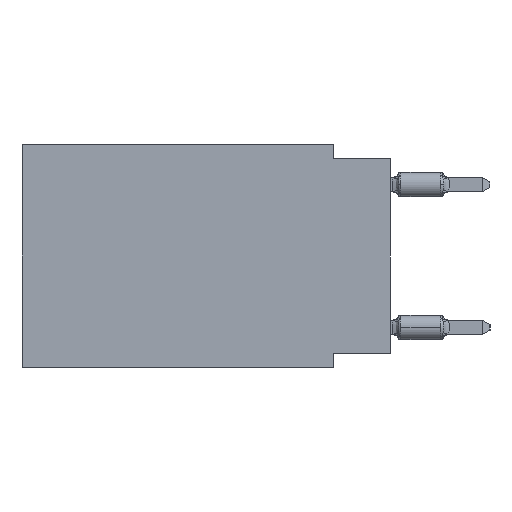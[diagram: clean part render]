
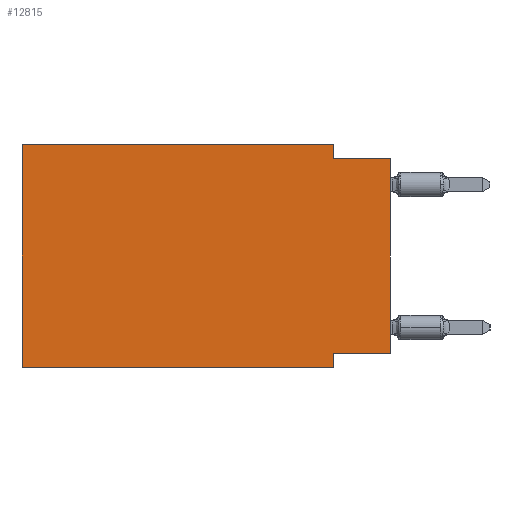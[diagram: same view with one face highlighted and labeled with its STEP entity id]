
A CAD part, left-side view. The second image highlights one B-rep face of the part: STEP entity #12815.
In plain terms, the highlighted planar face has unit normal (-1, 0, 0).
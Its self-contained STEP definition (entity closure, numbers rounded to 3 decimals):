
#8 = LINE ( 'NONE', #27565, #25493 ) ;
#121 = CARTESIAN_POINT ( 'NONE',  ( 0., 0., -0.635 ) ) ;
#505 = FACE_OUTER_BOUND ( 'NONE', #16886, .T. ) ;
#1928 = VERTEX_POINT ( 'NONE', #12826 ) ;
#2014 = VECTOR ( 'NONE', #6454, 1000. ) ;
#2536 = VECTOR ( 'NONE', #10480, 1000. ) ;
#2555 = DIRECTION ( 'NONE',  ( 0., 0., -1. ) ) ;
#2789 = EDGE_CURVE ( 'NONE', #16256, #33781, #26673, .T. ) ;
#3144 = CARTESIAN_POINT ( 'NONE',  ( 0., 2.54, -9.271 ) ) ;
#3362 = DIRECTION ( 'NONE',  ( 0., 0., -1. ) ) ;
#3942 = VECTOR ( 'NONE', #10360, 1000. ) ;
#4755 = ORIENTED_EDGE ( 'NONE', *, *, #26145, .F. ) ;
#4761 = VERTEX_POINT ( 'NONE', #11062 ) ;
#5014 = CARTESIAN_POINT ( 'NONE',  ( 0., 0., -0.635 ) ) ;
#6036 = VERTEX_POINT ( 'NONE', #17901 ) ;
#6356 = CARTESIAN_POINT ( 'NONE',  ( 0., 2.54, -0.635 ) ) ;
#6454 = DIRECTION ( 'NONE',  ( 0., 1., 0. ) ) ;
#7697 = EDGE_CURVE ( 'NONE', #24633, #19844, #32791, .T. ) ;
#9142 = LINE ( 'NONE', #11663, #2014 ) ;
#10360 = DIRECTION ( 'NONE',  ( 0., -1., 0. ) ) ;
#10480 = DIRECTION ( 'NONE',  ( 0., 0., -1. ) ) ;
#11062 = CARTESIAN_POINT ( 'NONE',  ( 0., 0., -9.271 ) ) ;
#11663 = CARTESIAN_POINT ( 'NONE',  ( 0., 0., -9.271 ) ) ;
#11963 = VERTEX_POINT ( 'NONE', #13525 ) ;
#12730 = DIRECTION ( 'NONE',  ( 0., 0., 1. ) ) ;
#12815 = ADVANCED_FACE ( 'NONE', ( #505 ), #17129, .F. ) ;
#12826 = CARTESIAN_POINT ( 'NONE',  ( 0., 16.383, -9.906 ) ) ;
#13525 = CARTESIAN_POINT ( 'NONE',  ( 0., 16.383, 0. ) ) ;
#14263 = CARTESIAN_POINT ( 'NONE',  ( 0., 16.383, 0. ) ) ;
#15282 = CARTESIAN_POINT ( 'NONE',  ( 0., 16.383, 0. ) ) ;
#15452 = DIRECTION ( 'NONE',  ( 0., -1., 0. ) ) ;
#15518 = ORIENTED_EDGE ( 'NONE', *, *, #23093, .F. ) ;
#16256 = VERTEX_POINT ( 'NONE', #6356 ) ;
#16886 = EDGE_LOOP ( 'NONE', ( #29192, #31551, #15518, #4755, #21598, #26963, #17362, #29171 ) ) ;
#17129 = PLANE ( 'NONE',  #26998 ) ;
#17362 = ORIENTED_EDGE ( 'NONE', *, *, #7697, .F. ) ;
#17901 = CARTESIAN_POINT ( 'NONE',  ( 0., 2.54, 0. ) ) ;
#18662 = CARTESIAN_POINT ( 'NONE',  ( 0., 16.383, 0. ) ) ;
#19340 = VECTOR ( 'NONE', #22063, 1000. ) ;
#19599 = EDGE_CURVE ( 'NONE', #4761, #24633, #9142, .T. ) ;
#19844 = VERTEX_POINT ( 'NONE', #29571 ) ;
#20616 = LINE ( 'NONE', #18662, #23192 ) ;
#21357 = LINE ( 'NONE', #15282, #27775 ) ;
#21598 = ORIENTED_EDGE ( 'NONE', *, *, #26578, .F. ) ;
#21619 = LINE ( 'NONE', #29491, #2536 ) ;
#22063 = DIRECTION ( 'NONE',  ( 0., -1., 0. ) ) ;
#23093 = EDGE_CURVE ( 'NONE', #6036, #16256, #21619, .T. ) ;
#23192 = VECTOR ( 'NONE', #12730, 1000. ) ;
#24412 = CARTESIAN_POINT ( 'NONE',  ( 0., 2.54, -9.906 ) ) ;
#24577 = CARTESIAN_POINT ( 'NONE',  ( 0., 16.383, -9.906 ) ) ;
#24633 = VERTEX_POINT ( 'NONE', #3144 ) ;
#25264 = LINE ( 'NONE', #24577, #19340 ) ;
#25493 = VECTOR ( 'NONE', #33134, 1000. ) ;
#26145 = EDGE_CURVE ( 'NONE', #11963, #6036, #21357, .T. ) ;
#26199 = VECTOR ( 'NONE', #2555, 1000. ) ;
#26578 = EDGE_CURVE ( 'NONE', #1928, #11963, #20616, .T. ) ;
#26673 = LINE ( 'NONE', #5014, #3942 ) ;
#26963 = ORIENTED_EDGE ( 'NONE', *, *, #30927, .T. ) ;
#26998 = AXIS2_PLACEMENT_3D ( 'NONE', #14263, #28036, #3362 ) ;
#27565 = CARTESIAN_POINT ( 'NONE',  ( 0., 0., 0. ) ) ;
#27775 = VECTOR ( 'NONE', #15452, 1000. ) ;
#28036 = DIRECTION ( 'NONE',  ( 1., 0., 0. ) ) ;
#28716 = EDGE_CURVE ( 'NONE', #4761, #33781, #8, .T. ) ;
#29171 = ORIENTED_EDGE ( 'NONE', *, *, #19599, .F. ) ;
#29192 = ORIENTED_EDGE ( 'NONE', *, *, #28716, .T. ) ;
#29491 = CARTESIAN_POINT ( 'NONE',  ( 0., 2.54, 0. ) ) ;
#29571 = CARTESIAN_POINT ( 'NONE',  ( 0., 2.54, -9.906 ) ) ;
#30927 = EDGE_CURVE ( 'NONE', #1928, #19844, #25264, .T. ) ;
#31551 = ORIENTED_EDGE ( 'NONE', *, *, #2789, .F. ) ;
#32791 = LINE ( 'NONE', #24412, #26199 ) ;
#33134 = DIRECTION ( 'NONE',  ( 0., 0., 1. ) ) ;
#33781 = VERTEX_POINT ( 'NONE', #121 ) ;
